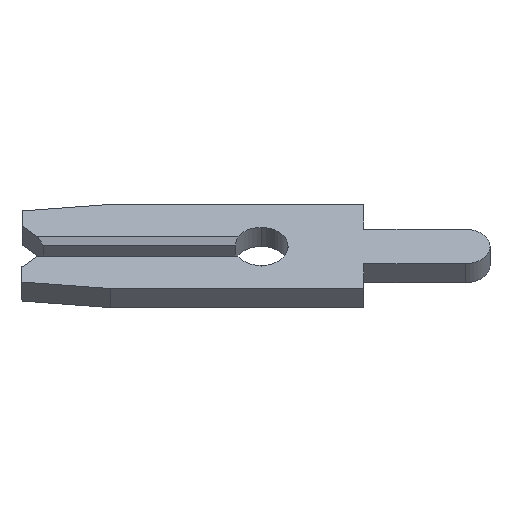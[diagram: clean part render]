
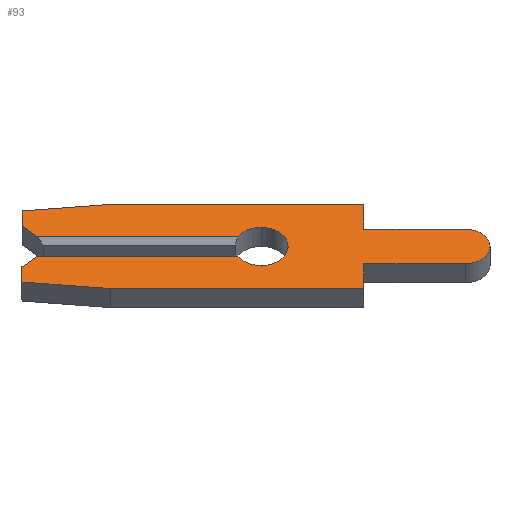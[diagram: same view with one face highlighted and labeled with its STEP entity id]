
A CAD part, left-side view. The second image highlights one B-rep face of the part: STEP entity #93.
In plain terms, the highlighted face is planar.
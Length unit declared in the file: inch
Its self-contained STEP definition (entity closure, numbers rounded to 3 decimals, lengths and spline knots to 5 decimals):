
#24 = EDGE_CURVE ( 'NONE', #732, #32, #1018, .T. ) ;
#28 = VERTEX_POINT ( 'NONE', #384 ) ;
#32 = VERTEX_POINT ( 'NONE', #610 ) ;
#33 = CARTESIAN_POINT ( 'NONE',  ( -0.013, 0.231, 0.013 ) ) ;
#47 = CARTESIAN_POINT ( 'NONE',  ( -0.013, 0.2105, -0.0075 ) ) ;
#53 = DIRECTION ( 'NONE',  ( 0., 0.995, 0.105 ) ) ;
#66 = DIRECTION ( 'NONE',  ( -1., 0., 0. ) ) ;
#68 = VECTOR ( 'NONE', #345, 39.37008 ) ;
#70 = ORIENTED_EDGE ( 'NONE', *, *, #951, .F. ) ;
#93 = ADVANCED_FACE ( 'NONE', ( #419 ), #696, .F. ) ;
#98 = ORIENTED_EDGE ( 'NONE', *, *, #678, .T. ) ;
#110 = DIRECTION ( 'NONE',  ( -1., 0., 0. ) ) ;
#112 = CARTESIAN_POINT ( 'NONE',  ( -0.013, -0.1975, -0.0235 ) ) ;
#113 = LINE ( 'NONE', #33, #935 ) ;
#114 = LINE ( 'NONE', #151, #380 ) ;
#117 = DIRECTION ( 'NONE',  ( 0., 0., -1. ) ) ;
#122 = CARTESIAN_POINT ( 'NONE',  ( -0.013, 0., 0.026 ) ) ;
#133 = VERTEX_POINT ( 'NONE', #136 ) ;
#136 = CARTESIAN_POINT ( 'NONE',  ( -0.013, 0.02252, -0.013 ) ) ;
#138 = EDGE_CURVE ( 'NONE', #420, #288, #907, .T. ) ;
#148 = VECTOR ( 'NONE', #765, 39.37008 ) ;
#151 = CARTESIAN_POINT ( 'NONE',  ( -0.013, 0.146, -0.0575 ) ) ;
#165 = CARTESIAN_POINT ( 'NONE',  ( -0.013, 0.216, 0.013 ) ) ;
#172 = VECTOR ( 'NONE', #298, 39.37008 ) ;
#193 = AXIS2_PLACEMENT_3D ( 'NONE', #926, #66, #481 ) ;
#206 = ORIENTED_EDGE ( 'NONE', *, *, #276, .F. ) ;
#215 = VECTOR ( 'NONE', #1019, 39.37008 ) ;
#221 = CARTESIAN_POINT ( 'NONE',  ( -0.013, 0.231, 0.04857 ) ) ;
#228 = LINE ( 'NONE', #271, #68 ) ;
#271 = CARTESIAN_POINT ( 'NONE',  ( -0.013, -0.099, -0.0235 ) ) ;
#276 = EDGE_CURVE ( 'NONE', #490, #967, #114, .T. ) ;
#279 = DIRECTION ( 'NONE',  ( 0., 0., -1. ) ) ;
#284 = DIRECTION ( 'NONE',  ( 0., 0., 1. ) ) ;
#288 = VERTEX_POINT ( 'NONE', #777 ) ;
#297 = VERTEX_POINT ( 'NONE', #704 ) ;
#298 = DIRECTION ( 'NONE',  ( 0., 0., 1. ) ) ;
#310 = DIRECTION ( 'NONE',  ( 0., -0.995, 0.105 ) ) ;
#321 = EDGE_CURVE ( 'NONE', #288, #744, #476, .T. ) ;
#323 = CARTESIAN_POINT ( 'NONE',  ( -0.013, 0.146, -0.0575 ) ) ;
#326 = CIRCLE ( 'NONE', #358, 0.026 ) ;
#327 = VERTEX_POINT ( 'NONE', #165 ) ;
#336 = VECTOR ( 'NONE', #117, 39.37008 ) ;
#345 = DIRECTION ( 'NONE',  ( 0., 1., 0. ) ) ;
#354 = VECTOR ( 'NONE', #310, 39.37008 ) ;
#355 = ORIENTED_EDGE ( 'NONE', *, *, #833, .F. ) ;
#358 = AXIS2_PLACEMENT_3D ( 'NONE', #544, #548, #864 ) ;
#363 = EDGE_CURVE ( 'NONE', #606, #490, #892, .T. ) ;
#365 = DIRECTION ( 'NONE',  ( 0., 0.707, 0.707 ) ) ;
#380 = VECTOR ( 'NONE', #401, 39.37008 ) ;
#384 = CARTESIAN_POINT ( 'NONE',  ( -0.013, 0., -0.026 ) ) ;
#396 = ORIENTED_EDGE ( 'NONE', *, *, #909, .F. ) ;
#401 = DIRECTION ( 'NONE',  ( 0., 1., 0. ) ) ;
#407 = LINE ( 'NONE', #697, #172 ) ;
#419 = FACE_OUTER_BOUND ( 'NONE', #1027, .T. ) ;
#420 = VERTEX_POINT ( 'NONE', #804 ) ;
#423 = VECTOR ( 'NONE', #559, 39.37008 ) ;
#445 = CIRCLE ( 'NONE', #193, 0.026 ) ;
#463 = DIRECTION ( 'NONE',  ( 0., 0., -1. ) ) ;
#464 = VECTOR ( 'NONE', #791, 39.37008 ) ;
#467 = ORIENTED_EDGE ( 'NONE', *, *, #363, .F. ) ;
#470 = VERTEX_POINT ( 'NONE', #743 ) ;
#474 = LINE ( 'NONE', #676, #336 ) ;
#476 = LINE ( 'NONE', #494, #423 ) ;
#481 = DIRECTION ( 'NONE',  ( 0., 0., -1. ) ) ;
#488 = VERTEX_POINT ( 'NONE', #582 ) ;
#490 = VERTEX_POINT ( 'NONE', #657 ) ;
#494 = CARTESIAN_POINT ( 'NONE',  ( -0.013, 0.146, 0.0575 ) ) ;
#497 = LINE ( 'NONE', #912, #682 ) ;
#502 = CARTESIAN_POINT ( 'NONE',  ( -0.013, 0.231, -0.04857 ) ) ;
#503 = ORIENTED_EDGE ( 'NONE', *, *, #531, .F. ) ;
#514 = ORIENTED_EDGE ( 'NONE', *, *, #636, .F. ) ;
#524 = CIRCLE ( 'NONE', #590, 0.026 ) ;
#528 = ORIENTED_EDGE ( 'NONE', *, *, #888, .F. ) ;
#530 = ORIENTED_EDGE ( 'NONE', *, *, #138, .F. ) ;
#531 = EDGE_CURVE ( 'NONE', #700, #606, #228, .T. ) ;
#541 = LINE ( 'NONE', #714, #464 ) ;
#543 = VERTEX_POINT ( 'NONE', #502 ) ;
#544 = CARTESIAN_POINT ( 'NONE',  ( -0.013, 0., 0. ) ) ;
#548 = DIRECTION ( 'NONE',  ( -1., 0., 0. ) ) ;
#555 = VECTOR ( 'NONE', #53, 39.37008 ) ;
#559 = DIRECTION ( 'NONE',  ( 0., -1., 0. ) ) ;
#561 = AXIS2_PLACEMENT_3D ( 'NONE', #928, #601, #463 ) ;
#562 = CARTESIAN_POINT ( 'NONE',  ( -0.013, -0.099, -0.0575 ) ) ;
#582 = CARTESIAN_POINT ( 'NONE',  ( -0.013, -0.099, 0.0235 ) ) ;
#590 = AXIS2_PLACEMENT_3D ( 'NONE', #599, #110, #279 ) ;
#599 = CARTESIAN_POINT ( 'NONE',  ( -0.013, 0., 0. ) ) ;
#601 = DIRECTION ( 'NONE',  ( 1., 0., 0. ) ) ;
#604 = CARTESIAN_POINT ( 'NONE',  ( -0.013, 0.2105, 0.0075 ) ) ;
#606 = VERTEX_POINT ( 'NONE', #759 ) ;
#610 = CARTESIAN_POINT ( 'NONE',  ( -0.013, 0.216, -0.013 ) ) ;
#632 = VERTEX_POINT ( 'NONE', #122 ) ;
#636 = EDGE_CURVE ( 'NONE', #470, #700, #1025, .T. ) ;
#644 = LINE ( 'NONE', #604, #1012 ) ;
#657 = CARTESIAN_POINT ( 'NONE',  ( -0.013, -0.099, -0.0575 ) ) ;
#675 = ORIENTED_EDGE ( 'NONE', *, *, #747, .F. ) ;
#676 = CARTESIAN_POINT ( 'NONE',  ( -0.013, -0.099, 0.0575 ) ) ;
#678 = EDGE_CURVE ( 'NONE', #327, #779, #113, .T. ) ;
#682 = VECTOR ( 'NONE', #982, 39.37008 ) ;
#687 = ORIENTED_EDGE ( 'NONE', *, *, #987, .F. ) ;
#688 = CARTESIAN_POINT ( 'NONE',  ( -0.013, -0.1975, 0. ) ) ;
#693 = EDGE_CURVE ( 'NONE', #133, #28, #524, .T. ) ;
#696 = PLANE ( 'NONE',  #561 ) ;
#697 = CARTESIAN_POINT ( 'NONE',  ( -0.013, 0.231, 0.028 ) ) ;
#700 = VERTEX_POINT ( 'NONE', #112 ) ;
#704 = CARTESIAN_POINT ( 'NONE',  ( -0.013, 0.231, 0.028 ) ) ;
#708 = EDGE_CURVE ( 'NONE', #327, #297, #644, .T. ) ;
#711 = ORIENTED_EDGE ( 'NONE', *, *, #708, .F. ) ;
#714 = CARTESIAN_POINT ( 'NONE',  ( -0.013, 0., -0.013 ) ) ;
#720 = ORIENTED_EDGE ( 'NONE', *, *, #761, .F. ) ;
#732 = VERTEX_POINT ( 'NONE', #836 ) ;
#743 = CARTESIAN_POINT ( 'NONE',  ( -0.013, -0.1975, 0.0235 ) ) ;
#744 = VERTEX_POINT ( 'NONE', #838 ) ;
#747 = EDGE_CURVE ( 'NONE', #744, #488, #474, .T. ) ;
#759 = CARTESIAN_POINT ( 'NONE',  ( -0.013, -0.099, -0.0235 ) ) ;
#761 = EDGE_CURVE ( 'NONE', #488, #470, #497, .T. ) ;
#763 = DIRECTION ( 'NONE',  ( 0., -1., 0. ) ) ;
#765 = DIRECTION ( 'NONE',  ( 0., -0.707, 0.707 ) ) ;
#777 = CARTESIAN_POINT ( 'NONE',  ( -0.013, 0.146, 0.0575 ) ) ;
#779 = VERTEX_POINT ( 'NONE', #853 ) ;
#791 = DIRECTION ( 'NONE',  ( 0., -1., 0. ) ) ;
#793 = ORIENTED_EDGE ( 'NONE', *, *, #693, .F. ) ;
#804 = CARTESIAN_POINT ( 'NONE',  ( -0.013, 0.231, 0.04857 ) ) ;
#827 = LINE ( 'NONE', #937, #215 ) ;
#833 = EDGE_CURVE ( 'NONE', #297, #420, #407, .T. ) ;
#836 = CARTESIAN_POINT ( 'NONE',  ( -0.013, 0.231, -0.028 ) ) ;
#838 = CARTESIAN_POINT ( 'NONE',  ( -0.013, -0.099, 0.0575 ) ) ;
#846 = EDGE_CURVE ( 'NONE', #967, #543, #984, .T. ) ;
#853 = CARTESIAN_POINT ( 'NONE',  ( -0.013, 0.02252, 0.013 ) ) ;
#864 = DIRECTION ( 'NONE',  ( 0., 0., -1. ) ) ;
#866 = VECTOR ( 'NONE', #1036, 39.37008 ) ;
#879 = AXIS2_PLACEMENT_3D ( 'NONE', #688, #985, #284 ) ;
#885 = ORIENTED_EDGE ( 'NONE', *, *, #321, .F. ) ;
#888 = EDGE_CURVE ( 'NONE', #28, #632, #445, .T. ) ;
#892 = LINE ( 'NONE', #562, #866 ) ;
#907 = LINE ( 'NONE', #221, #354 ) ;
#909 = EDGE_CURVE ( 'NONE', #632, #779, #326, .T. ) ;
#912 = CARTESIAN_POINT ( 'NONE',  ( -0.013, -0.099, 0.0235 ) ) ;
#926 = CARTESIAN_POINT ( 'NONE',  ( -0.013, 0., 0. ) ) ;
#928 = CARTESIAN_POINT ( 'NONE',  ( -0.013, 0., 0. ) ) ;
#935 = VECTOR ( 'NONE', #763, 39.37008 ) ;
#937 = CARTESIAN_POINT ( 'NONE',  ( -0.013, 0.231, -0.028 ) ) ;
#951 = EDGE_CURVE ( 'NONE', #32, #133, #541, .T. ) ;
#967 = VERTEX_POINT ( 'NONE', #323 ) ;
#976 = ORIENTED_EDGE ( 'NONE', *, *, #24, .F. ) ;
#982 = DIRECTION ( 'NONE',  ( 0., -1., 0. ) ) ;
#984 = LINE ( 'NONE', #998, #555 ) ;
#985 = DIRECTION ( 'NONE',  ( 1., 0., 0. ) ) ;
#987 = EDGE_CURVE ( 'NONE', #543, #732, #827, .T. ) ;
#998 = CARTESIAN_POINT ( 'NONE',  ( -0.013, 0.231, -0.04857 ) ) ;
#1012 = VECTOR ( 'NONE', #365, 39.37008 ) ;
#1018 = LINE ( 'NONE', #47, #148 ) ;
#1019 = DIRECTION ( 'NONE',  ( 0., 0., 1. ) ) ;
#1025 = CIRCLE ( 'NONE', #879, 0.0235 ) ;
#1027 = EDGE_LOOP ( 'NONE', ( #98, #396, #528, #793, #70, #976, #687, #1029, #206, #467, #503, #514, #720, #675, #885, #530, #355, #711 ) ) ;
#1029 = ORIENTED_EDGE ( 'NONE', *, *, #846, .F. ) ;
#1036 = DIRECTION ( 'NONE',  ( 0., 0., -1. ) ) ;
